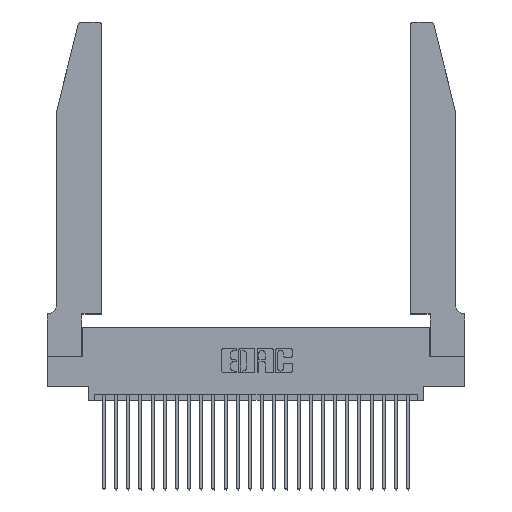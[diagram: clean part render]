
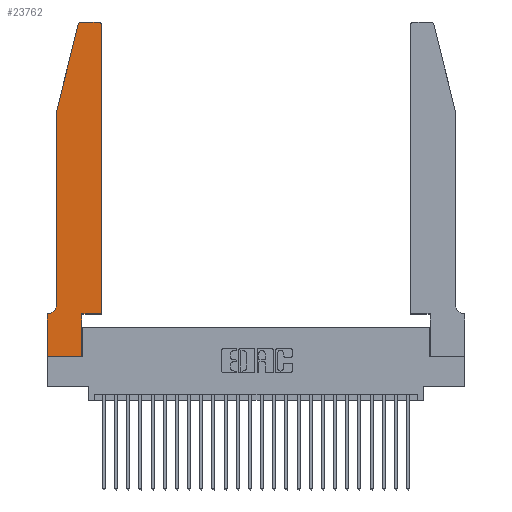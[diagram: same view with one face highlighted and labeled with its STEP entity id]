
A CAD part, top view. The second image highlights one B-rep face of the part: STEP entity #23762.
In plain terms, the highlighted planar face has unit normal (0, 0, 1).
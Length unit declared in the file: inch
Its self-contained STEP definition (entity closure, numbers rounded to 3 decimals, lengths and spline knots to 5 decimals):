
#602 = CARTESIAN_POINT ( 'NONE',  ( 0.284, 2.75, 0.37 ) ) ;
#958 = CARTESIAN_POINT ( 'NONE',  ( 0., 0.35, 0.37 ) ) ;
#996 = CARTESIAN_POINT ( 'NONE',  ( 0.2865, 0., 0.37 ) ) ;
#2038 = ORIENTED_EDGE ( 'NONE', *, *, #2968, .T. ) ;
#2187 = DIRECTION ( 'NONE',  ( 0., 1., 0. ) ) ;
#2226 = ORIENTED_EDGE ( 'NONE', *, *, #19482, .T. ) ;
#2421 = DIRECTION ( 'NONE',  ( 0., 0., 1. ) ) ;
#2770 = AXIS2_PLACEMENT_3D ( 'NONE', #6407, #25290, #14727 ) ;
#2779 = LINE ( 'NONE', #21197, #24723 ) ;
#2873 = CARTESIAN_POINT ( 'NONE',  ( 0.4205, 2.72, 0.37 ) ) ;
#2968 = EDGE_CURVE ( 'NONE', #23119, #12326, #25762, .T. ) ;
#2977 = VERTEX_POINT ( 'NONE', #19748 ) ;
#3552 = FACE_OUTER_BOUND ( 'NONE', #26074, .T. ) ;
#3634 = CARTESIAN_POINT ( 'NONE',  ( 0.0055, 0.35, 0.37 ) ) ;
#3701 = LINE ( 'NONE', #24895, #22035 ) ;
#4135 = LINE ( 'NONE', #5308, #4772 ) ;
#4585 = CARTESIAN_POINT ( 'NONE',  ( 0.0755, 0.35, 0.37 ) ) ;
#4772 = VECTOR ( 'NONE', #22611, 39.37008 ) ;
#4945 = EDGE_CURVE ( 'NONE', #2977, #21085, #4135, .T. ) ;
#5106 = DIRECTION ( 'NONE',  ( 0., 0., 1. ) ) ;
#5308 = CARTESIAN_POINT ( 'NONE',  ( 0.2605, 2.75, 0.37 ) ) ;
#5762 = DIRECTION ( 'NONE',  ( 1., 0., 0. ) ) ;
#5812 = DIRECTION ( 'NONE',  ( 0., 1., 0. ) ) ;
#6407 = CARTESIAN_POINT ( 'NONE',  ( 0.0055, 0.42, 0.37 ) ) ;
#6681 = CARTESIAN_POINT ( 'NONE',  ( 0.284, 2.72, 0.37 ) ) ;
#6957 = AXIS2_PLACEMENT_3D ( 'NONE', #6681, #2421, #21950 ) ;
#7134 = CIRCLE ( 'NONE', #2770, 0.07 ) ;
#7164 = DIRECTION ( 'NONE',  ( 1., 0., 0. ) ) ;
#7439 = VERTEX_POINT ( 'NONE', #18423 ) ;
#7555 = DIRECTION ( 'NONE',  ( 0., 0., 1. ) ) ;
#7720 = ORIENTED_EDGE ( 'NONE', *, *, #13840, .T. ) ;
#8975 = LINE ( 'NONE', #24522, #27235 ) ;
#9427 = DIRECTION ( 'NONE',  ( 1., 0., 0. ) ) ;
#9923 = VERTEX_POINT ( 'NONE', #12041 ) ;
#10039 = LINE ( 'NONE', #15148, #26312 ) ;
#10118 = CARTESIAN_POINT ( 'NONE',  ( 0.4505, 0.35, 0.37 ) ) ;
#10534 = VERTEX_POINT ( 'NONE', #22795 ) ;
#10629 = EDGE_CURVE ( 'NONE', #9923, #23119, #7134, .T. ) ;
#10919 = DIRECTION ( 'NONE',  ( -1., 0., 0. ) ) ;
#11174 = EDGE_CURVE ( 'NONE', #12326, #7439, #2779, .T. ) ;
#11417 = EDGE_CURVE ( 'NONE', #23435, #9923, #24382, .T. ) ;
#11418 = ORIENTED_EDGE ( 'NONE', *, *, #16804, .T. ) ;
#12041 = CARTESIAN_POINT ( 'NONE',  ( 0.0755, 0.42, 0.37 ) ) ;
#12165 = DIRECTION ( 'NONE',  ( -0.239, -0.971, 0. ) ) ;
#12221 = EDGE_CURVE ( 'NONE', #15856, #27211, #10039, .T. ) ;
#12326 = VERTEX_POINT ( 'NONE', #19032 ) ;
#12504 = CARTESIAN_POINT ( 'NONE',  ( 0.0755, 2., 0.37 ) ) ;
#12565 = CARTESIAN_POINT ( 'NONE',  ( 0.4505, 2.72, 0.37 ) ) ;
#13430 = ORIENTED_EDGE ( 'NONE', *, *, #4945, .T. ) ;
#13690 = ORIENTED_EDGE ( 'NONE', *, *, #17091, .T. ) ;
#13721 = VERTEX_POINT ( 'NONE', #17970 ) ;
#13840 = EDGE_CURVE ( 'NONE', #7439, #15856, #8975, .T. ) ;
#13885 = CIRCLE ( 'NONE', #6957, 0.03 ) ;
#14468 = DIRECTION ( 'NONE',  ( 0., -1., 0. ) ) ;
#14727 = DIRECTION ( 'NONE',  ( -1., 0., 0. ) ) ;
#14764 = AXIS2_PLACEMENT_3D ( 'NONE', #958, #7555, #9427 ) ;
#14797 = ORIENTED_EDGE ( 'NONE', *, *, #19931, .T. ) ;
#15017 = VECTOR ( 'NONE', #5762, 39.37008 ) ;
#15106 = VECTOR ( 'NONE', #17578, 39.37008 ) ;
#15148 = CARTESIAN_POINT ( 'NONE',  ( 0.2865, 0.35, 0.37 ) ) ;
#15856 = VERTEX_POINT ( 'NONE', #996 ) ;
#16347 = ORIENTED_EDGE ( 'NONE', *, *, #11174, .T. ) ;
#16494 = VECTOR ( 'NONE', #10919, 39.37008 ) ;
#16804 = EDGE_CURVE ( 'NONE', #21085, #13721, #13885, .T. ) ;
#17091 = EDGE_CURVE ( 'NONE', #10534, #17618, #23826, .T. ) ;
#17578 = DIRECTION ( 'NONE',  ( 0., -1., 0. ) ) ;
#17618 = VERTEX_POINT ( 'NONE', #12565 ) ;
#17970 = CARTESIAN_POINT ( 'NONE',  ( 0.25487, 2.72718, 0.37 ) ) ;
#18339 = LINE ( 'NONE', #20600, #15017 ) ;
#18423 = CARTESIAN_POINT ( 'NONE',  ( 0., 0., 0.37 ) ) ;
#19032 = CARTESIAN_POINT ( 'NONE',  ( 0., 0.35, 0.37 ) ) ;
#19482 = EDGE_CURVE ( 'NONE', #17618, #2977, #20402, .T. ) ;
#19748 = CARTESIAN_POINT ( 'NONE',  ( 0.4205, 2.75, 0.37 ) ) ;
#19821 = CARTESIAN_POINT ( 'NONE',  ( 0.0755, 2., 0.37 ) ) ;
#19931 = EDGE_CURVE ( 'NONE', #13721, #23435, #3701, .T. ) ;
#20191 = DIRECTION ( 'NONE',  ( 1., 0., 0. ) ) ;
#20402 = CIRCLE ( 'NONE', #26926, 0.03 ) ;
#20600 = CARTESIAN_POINT ( 'NONE',  ( 0.4505, 0.35, 0.37 ) ) ;
#20881 = VECTOR ( 'NONE', #5812, 39.37008 ) ;
#21085 = VERTEX_POINT ( 'NONE', #602 ) ;
#21197 = CARTESIAN_POINT ( 'NONE',  ( 0., 0., 0.37 ) ) ;
#21235 = EDGE_CURVE ( 'NONE', #27211, #10534, #18339, .T. ) ;
#21950 = DIRECTION ( 'NONE',  ( 1., 0., 0. ) ) ;
#21974 = ORIENTED_EDGE ( 'NONE', *, *, #21235, .T. ) ;
#22035 = VECTOR ( 'NONE', #12165, 39.37008 ) ;
#22158 = ORIENTED_EDGE ( 'NONE', *, *, #11417, .T. ) ;
#22321 = ORIENTED_EDGE ( 'NONE', *, *, #10629, .T. ) ;
#22440 = ORIENTED_EDGE ( 'NONE', *, *, #12221, .T. ) ;
#22611 = DIRECTION ( 'NONE',  ( -1., 0., 0. ) ) ;
#22795 = CARTESIAN_POINT ( 'NONE',  ( 0.4505, 0.35, 0.37 ) ) ;
#23119 = VERTEX_POINT ( 'NONE', #3634 ) ;
#23435 = VERTEX_POINT ( 'NONE', #12504 ) ;
#23762 = ADVANCED_FACE ( 'NONE', ( #3552 ), #26317, .T. ) ;
#23826 = LINE ( 'NONE', #10118, #20881 ) ;
#24382 = LINE ( 'NONE', #19821, #15106 ) ;
#24499 = CARTESIAN_POINT ( 'NONE',  ( 0.2865, 0.35, 0.37 ) ) ;
#24522 = CARTESIAN_POINT ( 'NONE',  ( 0., 0., 0.37 ) ) ;
#24723 = VECTOR ( 'NONE', #14468, 39.37008 ) ;
#24895 = CARTESIAN_POINT ( 'NONE',  ( 0.0755, 2., 0.37 ) ) ;
#25290 = DIRECTION ( 'NONE',  ( 0., 0., -1. ) ) ;
#25762 = LINE ( 'NONE', #4585, #16494 ) ;
#26074 = EDGE_LOOP ( 'NONE', ( #13430, #11418, #14797, #22158, #22321, #2038, #16347, #7720, #22440, #21974, #13690, #2226 ) ) ;
#26312 = VECTOR ( 'NONE', #2187, 39.37008 ) ;
#26317 = PLANE ( 'NONE',  #14764 ) ;
#26926 = AXIS2_PLACEMENT_3D ( 'NONE', #2873, #5106, #7164 ) ;
#27211 = VERTEX_POINT ( 'NONE', #24499 ) ;
#27235 = VECTOR ( 'NONE', #20191, 39.37008 ) ;
